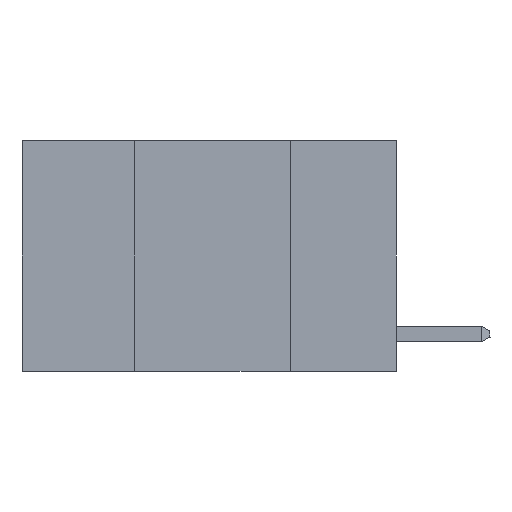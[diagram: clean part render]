
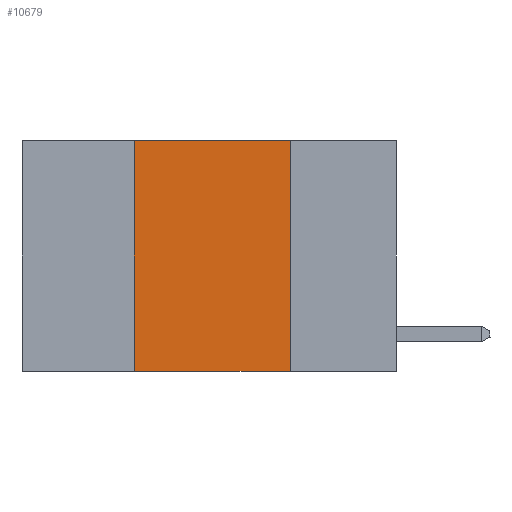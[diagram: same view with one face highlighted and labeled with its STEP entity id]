
A CAD part, left-side view. The second image highlights one B-rep face of the part: STEP entity #10679.
In plain terms, the highlighted planar face has unit normal (-1, 0, 0).
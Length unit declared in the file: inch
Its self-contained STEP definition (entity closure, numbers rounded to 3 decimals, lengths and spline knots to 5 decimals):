
#183 = VECTOR ( 'NONE', #13769, 39.37008 ) ;
#413 = CARTESIAN_POINT ( 'NONE',  ( 0., 0.17, 0. ) ) ;
#1574 = EDGE_LOOP ( 'NONE', ( #2916, #4094, #12123, #17247 ) ) ;
#1982 = LINE ( 'NONE', #413, #2450 ) ;
#2450 = VECTOR ( 'NONE', #11098, 39.37008 ) ;
#2729 = CARTESIAN_POINT ( 'NONE',  ( 0., 0.42, 0. ) ) ;
#2789 = VECTOR ( 'NONE', #4778, 39.37008 ) ;
#2876 = DIRECTION ( 'NONE',  ( 1., 0., 0. ) ) ;
#2916 = ORIENTED_EDGE ( 'NONE', *, *, #3322, .F. ) ;
#3322 = EDGE_CURVE ( 'NONE', #4153, #16084, #1982, .T. ) ;
#3858 = EDGE_CURVE ( 'NONE', #10279, #15147, #8123, .T. ) ;
#4094 = ORIENTED_EDGE ( 'NONE', *, *, #16062, .F. ) ;
#4153 = VERTEX_POINT ( 'NONE', #13016 ) ;
#4778 = DIRECTION ( 'NONE',  ( 0., -1., 0. ) ) ;
#5183 = FACE_OUTER_BOUND ( 'NONE', #1574, .T. ) ;
#6496 = CARTESIAN_POINT ( 'NONE',  ( 0., 0.42, -0.37 ) ) ;
#6660 = EDGE_CURVE ( 'NONE', #10279, #16084, #17036, .T. ) ;
#8123 = LINE ( 'NONE', #9133, #183 ) ;
#8991 = VECTOR ( 'NONE', #11860, 39.37008 ) ;
#9133 = CARTESIAN_POINT ( 'NONE',  ( 0., 0.42, 0. ) ) ;
#9472 = AXIS2_PLACEMENT_3D ( 'NONE', #12025, #2876, #13566 ) ;
#10279 = VERTEX_POINT ( 'NONE', #6496 ) ;
#10292 = CARTESIAN_POINT ( 'NONE',  ( 0., 0.6, -0.37 ) ) ;
#10679 = ADVANCED_FACE ( 'NONE', ( #5183 ), #18005, .F. ) ;
#11098 = DIRECTION ( 'NONE',  ( 0., 0., -1. ) ) ;
#11860 = DIRECTION ( 'NONE',  ( 0., -1., 0. ) ) ;
#12025 = CARTESIAN_POINT ( 'NONE',  ( 0., 0.6, 0. ) ) ;
#12123 = ORIENTED_EDGE ( 'NONE', *, *, #3858, .F. ) ;
#13016 = CARTESIAN_POINT ( 'NONE',  ( 0., 0.17, 0. ) ) ;
#13566 = DIRECTION ( 'NONE',  ( 0., 0., -1. ) ) ;
#13769 = DIRECTION ( 'NONE',  ( 0., 0., 1. ) ) ;
#14929 = LINE ( 'NONE', #15379, #2789 ) ;
#15147 = VERTEX_POINT ( 'NONE', #2729 ) ;
#15379 = CARTESIAN_POINT ( 'NONE',  ( 0., 0.6, 0. ) ) ;
#16062 = EDGE_CURVE ( 'NONE', #15147, #4153, #14929, .T. ) ;
#16084 = VERTEX_POINT ( 'NONE', #18473 ) ;
#17036 = LINE ( 'NONE', #10292, #8991 ) ;
#17247 = ORIENTED_EDGE ( 'NONE', *, *, #6660, .T. ) ;
#18005 = PLANE ( 'NONE',  #9472 ) ;
#18473 = CARTESIAN_POINT ( 'NONE',  ( 0., 0.17, -0.37 ) ) ;
